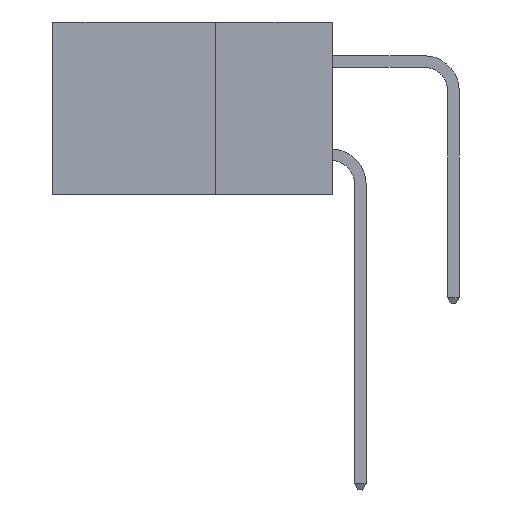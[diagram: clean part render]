
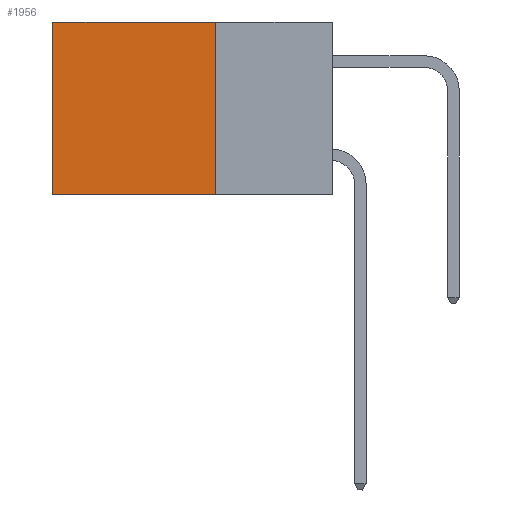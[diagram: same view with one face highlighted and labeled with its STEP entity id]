
A CAD part, left-side view. The second image highlights one B-rep face of the part: STEP entity #1956.
In plain terms, the highlighted planar face has unit normal (-1, 0, 0).
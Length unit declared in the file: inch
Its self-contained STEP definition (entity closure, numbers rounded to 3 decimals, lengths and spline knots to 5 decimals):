
#225 = CARTESIAN_POINT ( 'NONE',  ( 0.298, 0.6, -0.37 ) ) ;
#245 = AXIS2_PLACEMENT_3D ( 'NONE', #13817, #13697, #10849 ) ;
#349 = FACE_OUTER_BOUND ( 'NONE', #16171, .T. ) ;
#576 = PLANE ( 'NONE',  #245 ) ;
#980 = LINE ( 'NONE', #16463, #15559 ) ;
#1876 = VERTEX_POINT ( 'NONE', #225 ) ;
#1956 = ADVANCED_FACE ( 'NONE', ( #349 ), #576, .F. ) ;
#2094 = DIRECTION ( 'NONE',  ( 0., 1., 0. ) ) ;
#2138 = ORIENTED_EDGE ( 'NONE', *, *, #15044, .T. ) ;
#2709 = DIRECTION ( 'NONE',  ( 0., 0., -1. ) ) ;
#3665 = ORIENTED_EDGE ( 'NONE', *, *, #16331, .T. ) ;
#3886 = LINE ( 'NONE', #14589, #7332 ) ;
#4752 = VERTEX_POINT ( 'NONE', #6060 ) ;
#4896 = EDGE_CURVE ( 'NONE', #16376, #1876, #13434, .T. ) ;
#5983 = VERTEX_POINT ( 'NONE', #8178 ) ;
#6060 = CARTESIAN_POINT ( 'NONE',  ( 0.298, 0.6, 0. ) ) ;
#7332 = VECTOR ( 'NONE', #2709, 39.37008 ) ;
#8058 = EDGE_CURVE ( 'NONE', #5983, #16376, #980, .T. ) ;
#8178 = CARTESIAN_POINT ( 'NONE',  ( 0.298, 0.25, 0. ) ) ;
#9925 = ORIENTED_EDGE ( 'NONE', *, *, #8058, .F. ) ;
#10542 = VECTOR ( 'NONE', #18174, 39.37008 ) ;
#10849 = DIRECTION ( 'NONE',  ( 0., 0., -1. ) ) ;
#12067 = VECTOR ( 'NONE', #2094, 39.37008 ) ;
#12117 = CARTESIAN_POINT ( 'NONE',  ( 0.298, 0.25, -0.37 ) ) ;
#12375 = ORIENTED_EDGE ( 'NONE', *, *, #4896, .F. ) ;
#13434 = LINE ( 'NONE', #12117, #12067 ) ;
#13697 = DIRECTION ( 'NONE',  ( 1., 0., 0. ) ) ;
#13817 = CARTESIAN_POINT ( 'NONE',  ( 0.298, 0.25, 0. ) ) ;
#14589 = CARTESIAN_POINT ( 'NONE',  ( 0.298, 0.6, 0. ) ) ;
#15044 = EDGE_CURVE ( 'NONE', #4752, #1876, #3886, .T. ) ;
#15559 = VECTOR ( 'NONE', #17942, 39.37008 ) ;
#16171 = EDGE_LOOP ( 'NONE', ( #2138, #12375, #9925, #3665 ) ) ;
#16331 = EDGE_CURVE ( 'NONE', #5983, #4752, #18710, .T. ) ;
#16376 = VERTEX_POINT ( 'NONE', #18433 ) ;
#16463 = CARTESIAN_POINT ( 'NONE',  ( 0.298, 0.25, 0. ) ) ;
#16966 = CARTESIAN_POINT ( 'NONE',  ( 0.298, 0.25, 0. ) ) ;
#17942 = DIRECTION ( 'NONE',  ( 0., 0., -1. ) ) ;
#18174 = DIRECTION ( 'NONE',  ( 0., 1., 0. ) ) ;
#18433 = CARTESIAN_POINT ( 'NONE',  ( 0.298, 0.25, -0.37 ) ) ;
#18710 = LINE ( 'NONE', #16966, #10542 ) ;
